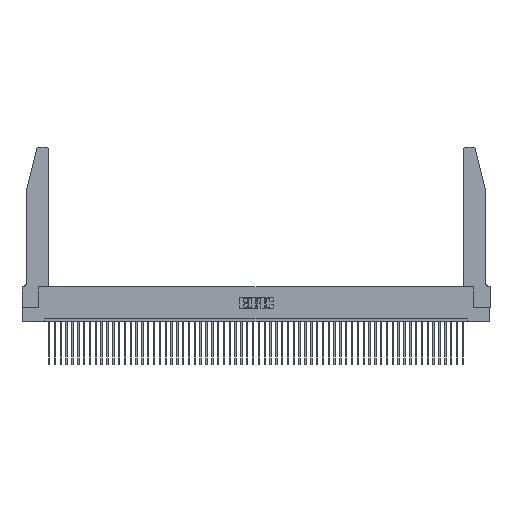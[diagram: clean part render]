
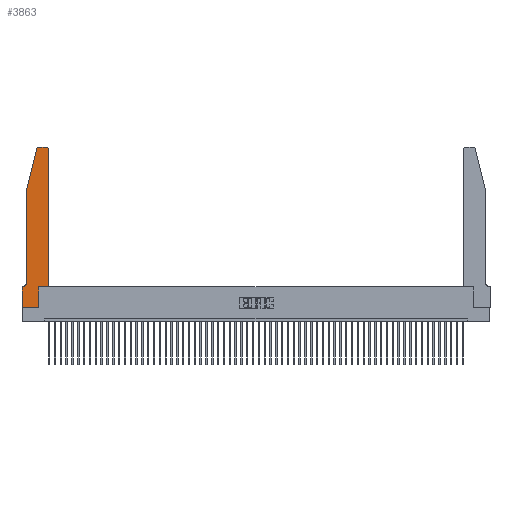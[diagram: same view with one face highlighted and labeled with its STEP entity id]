
A CAD part, top view. The second image highlights one B-rep face of the part: STEP entity #3863.
In plain terms, the highlighted planar face has unit normal (0, 0, 1).
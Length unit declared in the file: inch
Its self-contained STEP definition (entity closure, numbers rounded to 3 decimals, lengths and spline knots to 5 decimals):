
#119 = VECTOR ( 'NONE', #40724, 39.37008 ) ;
#1147 = LINE ( 'NONE', #33196, #27013 ) ;
#1204 = LINE ( 'NONE', #3849, #9822 ) ;
#3135 = AXIS2_PLACEMENT_3D ( 'NONE', #14185, #52377, #53659 ) ;
#3198 = EDGE_CURVE ( 'NONE', #37446, #36468, #42222, .T. ) ;
#3849 = CARTESIAN_POINT ( 'NONE',  ( 0., 0., 0.37 ) ) ;
#3863 = ADVANCED_FACE ( 'NONE', ( #4371 ), #39573, .T. ) ;
#3998 = VERTEX_POINT ( 'NONE', #6963 ) ;
#4004 = CIRCLE ( 'NONE', #30541, 0.03 ) ;
#4371 = FACE_OUTER_BOUND ( 'NONE', #40859, .T. ) ;
#5730 = DIRECTION ( 'NONE',  ( 0., 0., -1. ) ) ;
#5820 = CARTESIAN_POINT ( 'NONE',  ( 0.4505, 0.35, 0.37 ) ) ;
#6839 = CARTESIAN_POINT ( 'NONE',  ( 0.4505, 0.35, 0.37 ) ) ;
#6963 = CARTESIAN_POINT ( 'NONE',  ( 0.0755, 2., 0.37 ) ) ;
#7443 = ORIENTED_EDGE ( 'NONE', *, *, #44982, .T. ) ;
#9337 = CARTESIAN_POINT ( 'NONE',  ( 0.0755, 0.42, 0.37 ) ) ;
#9375 = EDGE_CURVE ( 'NONE', #45279, #43736, #43805, .T. ) ;
#9822 = VECTOR ( 'NONE', #21196, 39.37008 ) ;
#9844 = ORIENTED_EDGE ( 'NONE', *, *, #37244, .T. ) ;
#10501 = EDGE_CURVE ( 'NONE', #40597, #13454, #12523, .T. ) ;
#12523 = LINE ( 'NONE', #20043, #13164 ) ;
#13164 = VECTOR ( 'NONE', #33197, 39.37008 ) ;
#13454 = VERTEX_POINT ( 'NONE', #48546 ) ;
#14050 = CARTESIAN_POINT ( 'NONE',  ( 0.4505, 0.35, 0.37 ) ) ;
#14068 = CARTESIAN_POINT ( 'NONE',  ( 0.0055, 0.42, 0.37 ) ) ;
#14185 = CARTESIAN_POINT ( 'NONE',  ( 0., 0.35, 0.37 ) ) ;
#14826 = DIRECTION ( 'NONE',  ( -0.239, -0.971, 0. ) ) ;
#15600 = CARTESIAN_POINT ( 'NONE',  ( 0.284, 2.75, 0.37 ) ) ;
#16803 = CARTESIAN_POINT ( 'NONE',  ( 0., 0.35, 0.37 ) ) ;
#18253 = DIRECTION ( 'NONE',  ( 0., 1., 0. ) ) ;
#19436 = LINE ( 'NONE', #48034, #39360 ) ;
#19565 = CARTESIAN_POINT ( 'NONE',  ( 0.284, 2.72, 0.37 ) ) ;
#20043 = CARTESIAN_POINT ( 'NONE',  ( 0., 0., 0.37 ) ) ;
#20389 = DIRECTION ( 'NONE',  ( 1., 0., 0. ) ) ;
#20659 = AXIS2_PLACEMENT_3D ( 'NONE', #25227, #54714, #20389 ) ;
#20841 = CARTESIAN_POINT ( 'NONE',  ( 0.4505, 2.72, 0.37 ) ) ;
#21196 = DIRECTION ( 'NONE',  ( 1., 0., 0. ) ) ;
#21784 = VERTEX_POINT ( 'NONE', #5820 ) ;
#23312 = EDGE_CURVE ( 'NONE', #21784, #46163, #45674, .T. ) ;
#23450 = VERTEX_POINT ( 'NONE', #32142 ) ;
#25008 = CARTESIAN_POINT ( 'NONE',  ( 0.0755, 2., 0.37 ) ) ;
#25123 = ORIENTED_EDGE ( 'NONE', *, *, #49951, .T. ) ;
#25227 = CARTESIAN_POINT ( 'NONE',  ( 0.4205, 2.72, 0.37 ) ) ;
#27013 = VECTOR ( 'NONE', #28203, 39.37008 ) ;
#27215 = DIRECTION ( 'NONE',  ( -1., 0., 0. ) ) ;
#28203 = DIRECTION ( 'NONE',  ( -1., 0., 0. ) ) ;
#29212 = ORIENTED_EDGE ( 'NONE', *, *, #23312, .T. ) ;
#29233 = DIRECTION ( 'NONE',  ( 0., -1., 0. ) ) ;
#30541 = AXIS2_PLACEMENT_3D ( 'NONE', #19565, #32728, #40735 ) ;
#30899 = VERTEX_POINT ( 'NONE', #15600 ) ;
#30920 = VECTOR ( 'NONE', #47408, 39.37008 ) ;
#32142 = CARTESIAN_POINT ( 'NONE',  ( 0.25487, 2.72718, 0.37 ) ) ;
#32676 = LINE ( 'NONE', #35568, #33361 ) ;
#32728 = DIRECTION ( 'NONE',  ( 0., 0., 1. ) ) ;
#32799 = VERTEX_POINT ( 'NONE', #50295 ) ;
#33196 = CARTESIAN_POINT ( 'NONE',  ( 0.2605, 2.75, 0.37 ) ) ;
#33197 = DIRECTION ( 'NONE',  ( 0., -1., 0. ) ) ;
#33283 = ORIENTED_EDGE ( 'NONE', *, *, #10501, .T. ) ;
#33361 = VECTOR ( 'NONE', #14826, 39.37008 ) ;
#33415 = CIRCLE ( 'NONE', #20659, 0.03 ) ;
#33478 = EDGE_CURVE ( 'NONE', #3998, #45279, #33665, .T. ) ;
#33665 = LINE ( 'NONE', #25008, #50945 ) ;
#34234 = CARTESIAN_POINT ( 'NONE',  ( 0.2865, 0.35, 0.37 ) ) ;
#35568 = CARTESIAN_POINT ( 'NONE',  ( 0.0755, 2., 0.37 ) ) ;
#35948 = CARTESIAN_POINT ( 'NONE',  ( 0.2865, 0.35, 0.37 ) ) ;
#36468 = VERTEX_POINT ( 'NONE', #35948 ) ;
#36606 = AXIS2_PLACEMENT_3D ( 'NONE', #14068, #5730, #27215 ) ;
#37244 = EDGE_CURVE ( 'NONE', #36468, #21784, #53133, .T. ) ;
#37446 = VERTEX_POINT ( 'NONE', #46781 ) ;
#37764 = ORIENTED_EDGE ( 'NONE', *, *, #3198, .T. ) ;
#38575 = ORIENTED_EDGE ( 'NONE', *, *, #41989, .T. ) ;
#39360 = VECTOR ( 'NONE', #39498, 39.37008 ) ;
#39498 = DIRECTION ( 'NONE',  ( -1., 0., 0. ) ) ;
#39573 = PLANE ( 'NONE',  #3135 ) ;
#40597 = VERTEX_POINT ( 'NONE', #16803 ) ;
#40724 = DIRECTION ( 'NONE',  ( 1., 0., 0. ) ) ;
#40735 = DIRECTION ( 'NONE',  ( 1., 0., 0. ) ) ;
#40859 = EDGE_LOOP ( 'NONE', ( #7443, #25123, #38575, #53070, #45202, #51654, #33283, #48356, #37764, #9844, #29212, #45807 ) ) ;
#41691 = VECTOR ( 'NONE', #18253, 39.37008 ) ;
#41989 = EDGE_CURVE ( 'NONE', #23450, #3998, #32676, .T. ) ;
#42222 = LINE ( 'NONE', #34234, #30920 ) ;
#43736 = VERTEX_POINT ( 'NONE', #47459 ) ;
#43805 = CIRCLE ( 'NONE', #36606, 0.07 ) ;
#44494 = EDGE_CURVE ( 'NONE', #13454, #37446, #1204, .T. ) ;
#44982 = EDGE_CURVE ( 'NONE', #32799, #30899, #1147, .T. ) ;
#45202 = ORIENTED_EDGE ( 'NONE', *, *, #9375, .T. ) ;
#45279 = VERTEX_POINT ( 'NONE', #9337 ) ;
#45674 = LINE ( 'NONE', #14050, #41691 ) ;
#45807 = ORIENTED_EDGE ( 'NONE', *, *, #53938, .T. ) ;
#46163 = VERTEX_POINT ( 'NONE', #20841 ) ;
#46781 = CARTESIAN_POINT ( 'NONE',  ( 0.2865, 0., 0.37 ) ) ;
#47397 = EDGE_CURVE ( 'NONE', #43736, #40597, #19436, .T. ) ;
#47408 = DIRECTION ( 'NONE',  ( 0., 1., 0. ) ) ;
#47459 = CARTESIAN_POINT ( 'NONE',  ( 0.0055, 0.35, 0.37 ) ) ;
#48034 = CARTESIAN_POINT ( 'NONE',  ( 0.0755, 0.35, 0.37 ) ) ;
#48356 = ORIENTED_EDGE ( 'NONE', *, *, #44494, .T. ) ;
#48546 = CARTESIAN_POINT ( 'NONE',  ( 0., 0., 0.37 ) ) ;
#49951 = EDGE_CURVE ( 'NONE', #30899, #23450, #4004, .T. ) ;
#50295 = CARTESIAN_POINT ( 'NONE',  ( 0.4205, 2.75, 0.37 ) ) ;
#50945 = VECTOR ( 'NONE', #29233, 39.37008 ) ;
#51654 = ORIENTED_EDGE ( 'NONE', *, *, #47397, .T. ) ;
#52377 = DIRECTION ( 'NONE',  ( 0., 0., 1. ) ) ;
#53070 = ORIENTED_EDGE ( 'NONE', *, *, #33478, .T. ) ;
#53133 = LINE ( 'NONE', #6839, #119 ) ;
#53659 = DIRECTION ( 'NONE',  ( 1., 0., 0. ) ) ;
#53938 = EDGE_CURVE ( 'NONE', #46163, #32799, #33415, .T. ) ;
#54714 = DIRECTION ( 'NONE',  ( 0., 0., 1. ) ) ;
